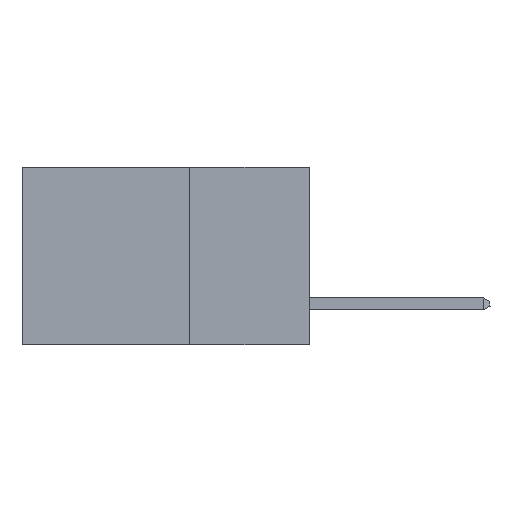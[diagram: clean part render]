
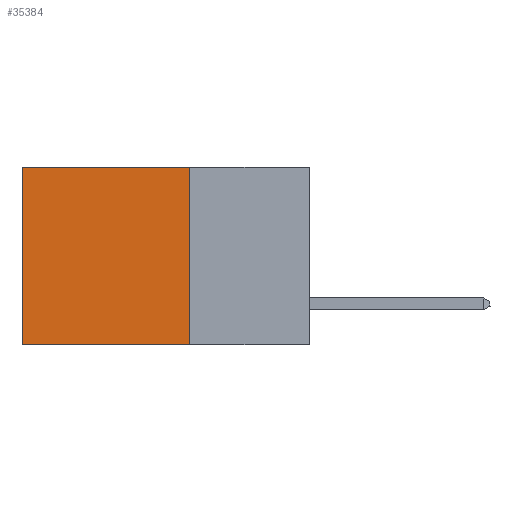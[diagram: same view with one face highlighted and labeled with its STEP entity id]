
A CAD part, left-side view. The second image highlights one B-rep face of the part: STEP entity #35384.
In plain terms, the highlighted planar face has unit normal (-1, 0, 0).
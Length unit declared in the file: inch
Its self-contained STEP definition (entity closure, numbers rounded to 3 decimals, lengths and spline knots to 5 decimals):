
#166 = VERTEX_POINT ( 'NONE', #33438 ) ;
#673 = LINE ( 'NONE', #27248, #30782 ) ;
#1020 = VERTEX_POINT ( 'NONE', #29447 ) ;
#2285 = EDGE_LOOP ( 'NONE', ( #10527, #35858, #33961, #28385 ) ) ;
#2752 = CARTESIAN_POINT ( 'NONE',  ( 0.2875, 0.25, 0. ) ) ;
#3276 = FACE_OUTER_BOUND ( 'NONE', #2285, .T. ) ;
#3901 = DIRECTION ( 'NONE',  ( 0., 1., 0. ) ) ;
#4745 = VECTOR ( 'NONE', #3901, 39.37008 ) ;
#4931 = EDGE_CURVE ( 'NONE', #1020, #166, #673, .T. ) ;
#5852 = VERTEX_POINT ( 'NONE', #34939 ) ;
#7238 = LINE ( 'NONE', #30735, #9505 ) ;
#7244 = DIRECTION ( 'NONE',  ( 0., 0., -1. ) ) ;
#7333 = CARTESIAN_POINT ( 'NONE',  ( 0.2875, 0.25, 0. ) ) ;
#9505 = VECTOR ( 'NONE', #19112, 39.37008 ) ;
#9709 = LINE ( 'NONE', #27298, #4745 ) ;
#10527 = ORIENTED_EDGE ( 'NONE', *, *, #4931, .T. ) ;
#10694 = CARTESIAN_POINT ( 'NONE',  ( 0.2875, 0.25, 0. ) ) ;
#13219 = EDGE_CURVE ( 'NONE', #29144, #1020, #7238, .T. ) ;
#14535 = DIRECTION ( 'NONE',  ( 0., 0., -1. ) ) ;
#15023 = EDGE_CURVE ( 'NONE', #29144, #5852, #30067, .T. ) ;
#17067 = DIRECTION ( 'NONE',  ( 1., 0., 0. ) ) ;
#19112 = DIRECTION ( 'NONE',  ( 0., 1., 0. ) ) ;
#20961 = VECTOR ( 'NONE', #14535, 39.37008 ) ;
#22442 = PLANE ( 'NONE',  #31634 ) ;
#27248 = CARTESIAN_POINT ( 'NONE',  ( 0.2875, 0.6, 0. ) ) ;
#27298 = CARTESIAN_POINT ( 'NONE',  ( 0.2875, 0.25, -0.37 ) ) ;
#27834 = EDGE_CURVE ( 'NONE', #5852, #166, #9709, .T. ) ;
#28385 = ORIENTED_EDGE ( 'NONE', *, *, #13219, .T. ) ;
#29144 = VERTEX_POINT ( 'NONE', #7333 ) ;
#29447 = CARTESIAN_POINT ( 'NONE',  ( 0.2875, 0.6, 0. ) ) ;
#30067 = LINE ( 'NONE', #2752, #20961 ) ;
#30735 = CARTESIAN_POINT ( 'NONE',  ( 0.2875, 0.25, 0. ) ) ;
#30782 = VECTOR ( 'NONE', #7244, 39.37008 ) ;
#31251 = DIRECTION ( 'NONE',  ( 0., 0., -1. ) ) ;
#31634 = AXIS2_PLACEMENT_3D ( 'NONE', #10694, #17067, #31251 ) ;
#33438 = CARTESIAN_POINT ( 'NONE',  ( 0.2875, 0.6, -0.37 ) ) ;
#33961 = ORIENTED_EDGE ( 'NONE', *, *, #15023, .F. ) ;
#34939 = CARTESIAN_POINT ( 'NONE',  ( 0.2875, 0.25, -0.37 ) ) ;
#35384 = ADVANCED_FACE ( 'NONE', ( #3276 ), #22442, .F. ) ;
#35858 = ORIENTED_EDGE ( 'NONE', *, *, #27834, .F. ) ;
